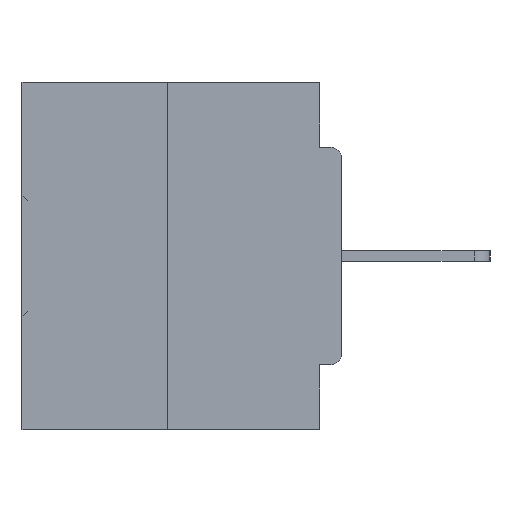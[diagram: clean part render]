
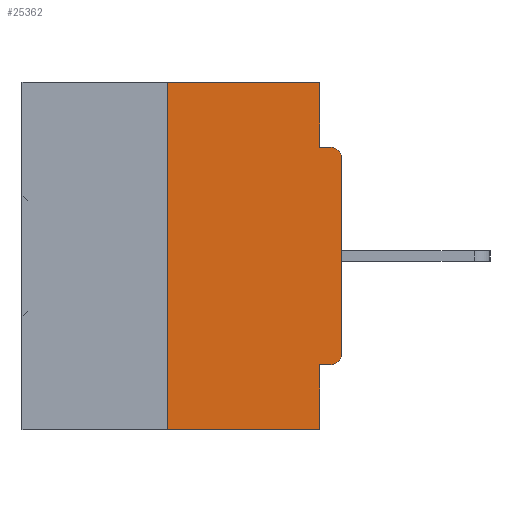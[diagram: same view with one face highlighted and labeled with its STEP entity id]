
A CAD part, left-side view. The second image highlights one B-rep face of the part: STEP entity #25362.
In plain terms, the highlighted planar face has unit normal (-1, 0, 0).
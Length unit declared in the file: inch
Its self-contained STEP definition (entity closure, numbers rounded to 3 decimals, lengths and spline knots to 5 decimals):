
#1195 = VERTEX_POINT ( 'NONE', #30563 ) ;
#1214 = VERTEX_POINT ( 'NONE', #2580 ) ;
#1626 = DIRECTION ( 'NONE',  ( 0., 0., 1. ) ) ;
#1876 = DIRECTION ( 'NONE',  ( 0., -1., 0. ) ) ;
#2097 = VERTEX_POINT ( 'NONE', #11252 ) ;
#2469 = CARTESIAN_POINT ( 'NONE',  ( 0., 0.031, 0. ) ) ;
#2580 = CARTESIAN_POINT ( 'NONE',  ( 0., 0.031, -0.0935 ) ) ;
#2626 = LINE ( 'NONE', #18710, #7289 ) ;
#2773 = VECTOR ( 'NONE', #39748, 39.37008 ) ;
#3018 = LINE ( 'NONE', #15608, #2773 ) ;
#3274 = DIRECTION ( 'NONE',  ( 0., 0., -1. ) ) ;
#3554 = LINE ( 'NONE', #22506, #17773 ) ;
#3665 = CARTESIAN_POINT ( 'NONE',  ( 0., 0.25, 0. ) ) ;
#3696 = VECTOR ( 'NONE', #22254, 39.37008 ) ;
#4179 = PLANE ( 'NONE',  #4902 ) ;
#4560 = ORIENTED_EDGE ( 'NONE', *, *, #39869, .T. ) ;
#4902 = AXIS2_PLACEMENT_3D ( 'NONE', #35209, #22321, #19654 ) ;
#6051 = DIRECTION ( 'NONE',  ( 0., 0., -1. ) ) ;
#6247 = VECTOR ( 'NONE', #6051, 39.37008 ) ;
#6973 = LINE ( 'NONE', #31091, #3696 ) ;
#7121 = VERTEX_POINT ( 'NONE', #24909 ) ;
#7289 = VECTOR ( 'NONE', #8533, 39.37008 ) ;
#8533 = DIRECTION ( 'NONE',  ( 0., -1., 0. ) ) ;
#10673 = FACE_OUTER_BOUND ( 'NONE', #18161, .T. ) ;
#10708 = EDGE_CURVE ( 'NONE', #1214, #26697, #14266, .T. ) ;
#11252 = CARTESIAN_POINT ( 'NONE',  ( 0., 0.031, -0.5 ) ) ;
#12335 = VERTEX_POINT ( 'NONE', #37226 ) ;
#12469 = AXIS2_PLACEMENT_3D ( 'NONE', #38198, #29028, #13052 ) ;
#12637 = VERTEX_POINT ( 'NONE', #3665 ) ;
#13052 = DIRECTION ( 'NONE',  ( 0., 0., -1. ) ) ;
#13197 = ORIENTED_EDGE ( 'NONE', *, *, #16762, .F. ) ;
#13872 = CARTESIAN_POINT ( 'NONE',  ( 0., 0., -0.0935 ) ) ;
#13990 = AXIS2_PLACEMENT_3D ( 'NONE', #15060, #40004, #3274 ) ;
#14266 = LINE ( 'NONE', #13872, #24702 ) ;
#15060 = CARTESIAN_POINT ( 'NONE',  ( 0., 0.015, -0.3915 ) ) ;
#15608 = CARTESIAN_POINT ( 'NONE',  ( 0., 0.031, 0. ) ) ;
#15929 = ORIENTED_EDGE ( 'NONE', *, *, #39538, .F. ) ;
#16134 = EDGE_CURVE ( 'NONE', #1195, #26697, #20302, .T. ) ;
#16762 = EDGE_CURVE ( 'NONE', #22091, #1214, #3018, .T. ) ;
#17266 = CARTESIAN_POINT ( 'NONE',  ( 0., 0.25, -0.5 ) ) ;
#17773 = VECTOR ( 'NONE', #28035, 39.37008 ) ;
#18073 = CARTESIAN_POINT ( 'NONE',  ( 0., 0., -0.3915 ) ) ;
#18161 = EDGE_LOOP ( 'NONE', ( #39525, #22106, #4560, #15929, #37520, #22370, #35585, #23215, #27466, #13197 ) ) ;
#18710 = CARTESIAN_POINT ( 'NONE',  ( 0., 0.46, 0. ) ) ;
#19654 = DIRECTION ( 'NONE',  ( 0., 0., -1. ) ) ;
#19941 = EDGE_CURVE ( 'NONE', #12637, #22091, #2626, .T. ) ;
#20302 = CIRCLE ( 'NONE', #12469, 0.015 ) ;
#20367 = LINE ( 'NONE', #29600, #39396 ) ;
#20902 = EDGE_CURVE ( 'NONE', #7121, #12335, #3554, .T. ) ;
#21212 = VERTEX_POINT ( 'NONE', #17266 ) ;
#21546 = CARTESIAN_POINT ( 'NONE',  ( 0., 0.031, -0.5 ) ) ;
#21958 = LINE ( 'NONE', #21546, #6247 ) ;
#22091 = VERTEX_POINT ( 'NONE', #2469 ) ;
#22106 = ORIENTED_EDGE ( 'NONE', *, *, #37682, .F. ) ;
#22254 = DIRECTION ( 'NONE',  ( 0., -1., 0. ) ) ;
#22321 = DIRECTION ( 'NONE',  ( 1., 0., 0. ) ) ;
#22370 = ORIENTED_EDGE ( 'NONE', *, *, #26112, .T. ) ;
#22506 = CARTESIAN_POINT ( 'NONE',  ( 0., 0., -0.4065 ) ) ;
#23215 = ORIENTED_EDGE ( 'NONE', *, *, #16134, .T. ) ;
#24702 = VECTOR ( 'NONE', #1876, 39.37008 ) ;
#24909 = CARTESIAN_POINT ( 'NONE',  ( 0., 0.015, -0.4065 ) ) ;
#24939 = LINE ( 'NONE', #31282, #27267 ) ;
#25362 = ADVANCED_FACE ( 'NONE', ( #10673 ), #4179, .F. ) ;
#26112 = EDGE_CURVE ( 'NONE', #7121, #35672, #31675, .T. ) ;
#26697 = VERTEX_POINT ( 'NONE', #29749 ) ;
#27267 = VECTOR ( 'NONE', #37389, 39.37008 ) ;
#27466 = ORIENTED_EDGE ( 'NONE', *, *, #10708, .F. ) ;
#28035 = DIRECTION ( 'NONE',  ( 0., 1., 0. ) ) ;
#29028 = DIRECTION ( 'NONE',  ( -1., 0., 0. ) ) ;
#29600 = CARTESIAN_POINT ( 'NONE',  ( 0., 0.25, 0. ) ) ;
#29749 = CARTESIAN_POINT ( 'NONE',  ( 0., 0.015, -0.0935 ) ) ;
#30563 = CARTESIAN_POINT ( 'NONE',  ( 0., 0., -0.1085 ) ) ;
#30649 = EDGE_CURVE ( 'NONE', #35672, #1195, #24939, .T. ) ;
#31091 = CARTESIAN_POINT ( 'NONE',  ( 0., 0.46, -0.5 ) ) ;
#31282 = CARTESIAN_POINT ( 'NONE',  ( 0., 0., 0. ) ) ;
#31675 = CIRCLE ( 'NONE', #13990, 0.015 ) ;
#35209 = CARTESIAN_POINT ( 'NONE',  ( 0., 0.46, 0. ) ) ;
#35585 = ORIENTED_EDGE ( 'NONE', *, *, #30649, .T. ) ;
#35672 = VERTEX_POINT ( 'NONE', #18073 ) ;
#37226 = CARTESIAN_POINT ( 'NONE',  ( 0., 0.031, -0.4065 ) ) ;
#37389 = DIRECTION ( 'NONE',  ( 0., 0., 1. ) ) ;
#37520 = ORIENTED_EDGE ( 'NONE', *, *, #20902, .F. ) ;
#37682 = EDGE_CURVE ( 'NONE', #21212, #12637, #20367, .T. ) ;
#38198 = CARTESIAN_POINT ( 'NONE',  ( 0., 0.015, -0.1085 ) ) ;
#39396 = VECTOR ( 'NONE', #1626, 39.37008 ) ;
#39525 = ORIENTED_EDGE ( 'NONE', *, *, #19941, .F. ) ;
#39538 = EDGE_CURVE ( 'NONE', #12335, #2097, #21958, .T. ) ;
#39748 = DIRECTION ( 'NONE',  ( 0., 0., -1. ) ) ;
#39869 = EDGE_CURVE ( 'NONE', #21212, #2097, #6973, .T. ) ;
#40004 = DIRECTION ( 'NONE',  ( -1., 0., 0. ) ) ;
